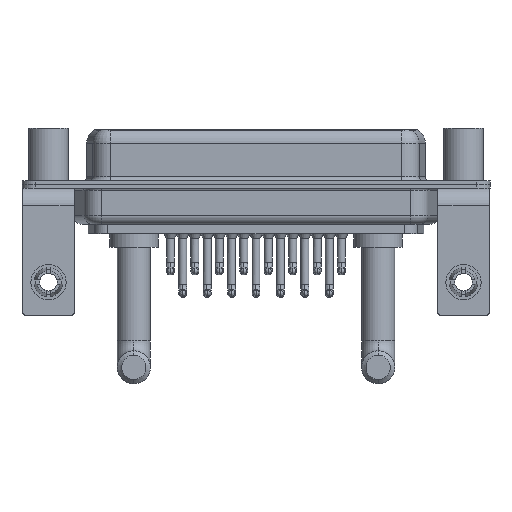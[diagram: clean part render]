
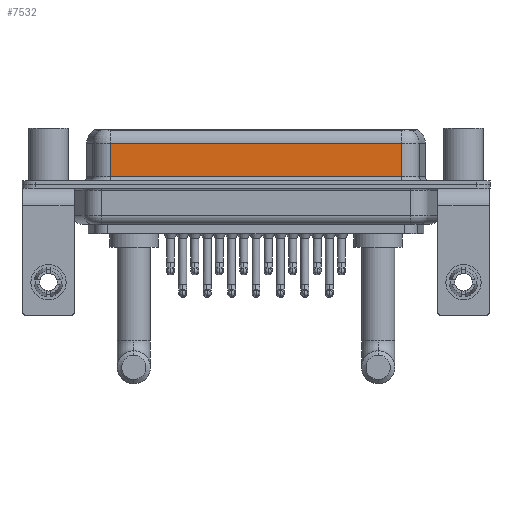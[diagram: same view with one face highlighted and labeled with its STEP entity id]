
A CAD part, front view. The second image highlights one B-rep face of the part: STEP entity #7532.
In plain terms, the highlighted planar face has unit normal (0, -1, 0).
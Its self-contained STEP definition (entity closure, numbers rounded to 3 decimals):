
#353 = VERTEX_POINT ( 'NONE', #13527 ) ;
#941 = ORIENTED_EDGE ( 'NONE', *, *, #20870, .F. ) ;
#1754 = CARTESIAN_POINT ( 'NONE',  ( 40.037, -3.95, 4.65 ) ) ;
#1996 = EDGE_LOOP ( 'NONE', ( #941, #13985, #18203, #11117 ) ) ;
#4974 = VECTOR ( 'NONE', #23963, 1000. ) ;
#5047 = CARTESIAN_POINT ( 'NONE',  ( 7.013, -3.95, 6.4 ) ) ;
#5737 = PLANE ( 'NONE',  #8853 ) ;
#6070 = DIRECTION ( 'NONE',  ( -1., 0., 0. ) ) ;
#6462 = VERTEX_POINT ( 'NONE', #9906 ) ;
#7395 = CARTESIAN_POINT ( 'NONE',  ( 40.037, -3.95, 6.4 ) ) ;
#7532 = ADVANCED_FACE ( 'NONE', ( #20990 ), #5737, .F. ) ;
#8342 = LINE ( 'NONE', #17801, #4974 ) ;
#8853 = AXIS2_PLACEMENT_3D ( 'NONE', #7395, #15366, #13225 ) ;
#9230 = LINE ( 'NONE', #5047, #14217 ) ;
#9906 = CARTESIAN_POINT ( 'NONE',  ( 40.037, -3.95, 0.9 ) ) ;
#10179 = CARTESIAN_POINT ( 'NONE',  ( 7.013, -3.95, 0.9 ) ) ;
#11117 = ORIENTED_EDGE ( 'NONE', *, *, #15087, .T. ) ;
#11118 = DIRECTION ( 'NONE',  ( 0., 0., -1. ) ) ;
#12349 = EDGE_CURVE ( 'NONE', #12990, #16381, #9230, .T. ) ;
#12703 = VECTOR ( 'NONE', #14814, 1000. ) ;
#12990 = VERTEX_POINT ( 'NONE', #13710 ) ;
#13225 = DIRECTION ( 'NONE',  ( 0., 0., 1. ) ) ;
#13527 = CARTESIAN_POINT ( 'NONE',  ( 40.037, -3.95, 4.65 ) ) ;
#13710 = CARTESIAN_POINT ( 'NONE',  ( 7.013, -3.95, 4.65 ) ) ;
#13985 = ORIENTED_EDGE ( 'NONE', *, *, #17098, .T. ) ;
#14217 = VECTOR ( 'NONE', #11118, 1000. ) ;
#14814 = DIRECTION ( 'NONE',  ( 1., 0., 0. ) ) ;
#15087 = EDGE_CURVE ( 'NONE', #16381, #6462, #16694, .T. ) ;
#15366 = DIRECTION ( 'NONE',  ( 0., 1., 0. ) ) ;
#16381 = VERTEX_POINT ( 'NONE', #10179 ) ;
#16694 = LINE ( 'NONE', #16814, #12703 ) ;
#16814 = CARTESIAN_POINT ( 'NONE',  ( 40.037, -3.95, 0.9 ) ) ;
#17098 = EDGE_CURVE ( 'NONE', #353, #12990, #22965, .T. ) ;
#17801 = CARTESIAN_POINT ( 'NONE',  ( 40.037, -3.95, 6.4 ) ) ;
#18203 = ORIENTED_EDGE ( 'NONE', *, *, #12349, .T. ) ;
#20870 = EDGE_CURVE ( 'NONE', #353, #6462, #8342, .T. ) ;
#20990 = FACE_OUTER_BOUND ( 'NONE', #1996, .T. ) ;
#22965 = LINE ( 'NONE', #1754, #24056 ) ;
#23963 = DIRECTION ( 'NONE',  ( 0., 0., -1. ) ) ;
#24056 = VECTOR ( 'NONE', #6070, 1000. ) ;
